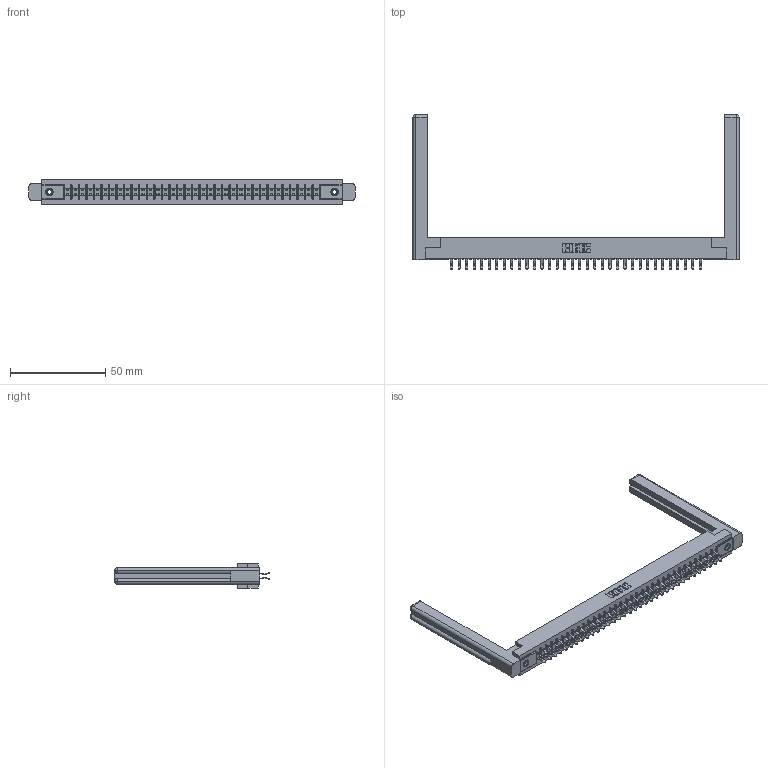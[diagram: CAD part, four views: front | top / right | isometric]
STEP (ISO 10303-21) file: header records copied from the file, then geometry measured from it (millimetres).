
FILE_DESCRIPTION (( 'STEP AP203' ), '1' );
FILE_NAME ('315-068-556-258.STEP', '2019-09-10T21:18:33', ( '' ), ( '' ), 'SwSTEP 2.0', 'SolidWorks 2016', '' );
FILE_SCHEMA (( 'CONFIG_CONTROL_DESIGN' ));
Length unit declared in the file: inch
Products named in the file (5): 315-068-556-258; 305-290-001_556; 305 Part_.156 Dia; 345-250-001_345-250-001-102; 307-220-058
Assembly tree (73 placements, depth 2):
  315-068-556-258
    305 Part_.156 Dia
    305-290-001_556  x68
    345-250-001_345-250-001-102  x2
    307-220-058  x2
Bounding box: 171.35 x 81.28 x 12.7 mm (x, y, z)
Volume: 24977.2 mm3; surface area: 27361.4 mm2
Topology: 73 solids, 73 shells, 4066 faces, 11652 edges, 7572 vertices
Faces by surface type: plane 2260, cylinder 1646, sphere 136, cone 12, torus 12
Entity records: 40642 total; most frequent: CARTESIAN_POINT 6743, ORIENTED_EDGE 6634, DIRECTION 6495, EDGE_CURVE 3317, LINE 2659, VECTOR 2659, VERTEX_POINT 2112, AXIS2_PLACEMENT_3D 1918
